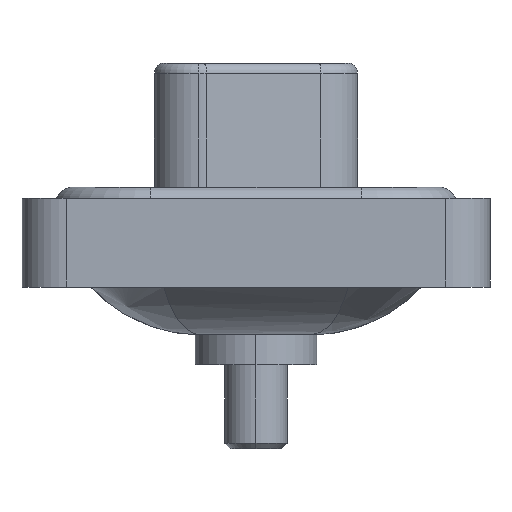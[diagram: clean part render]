
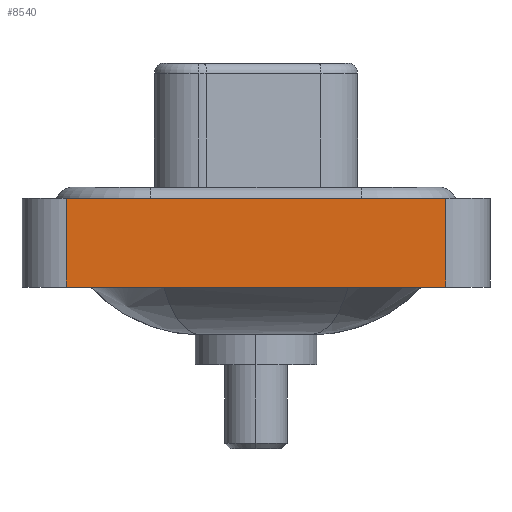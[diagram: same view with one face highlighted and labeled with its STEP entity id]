
A CAD part, left-side view. The second image highlights one B-rep face of the part: STEP entity #8540.
In plain terms, the highlighted planar face has unit normal (-1, 0, 0).
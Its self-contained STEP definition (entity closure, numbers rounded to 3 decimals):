
#223 = EDGE_LOOP ( 'NONE', ( #12306, #4261, #14064, #13628 ) ) ;
#631 = DIRECTION ( 'NONE',  ( 0., 0., 1. ) ) ;
#706 = CARTESIAN_POINT ( 'NONE',  ( -7.3, -8.55, -3.6 ) ) ;
#1344 = VECTOR ( 'NONE', #3159, 1000. ) ;
#1601 = EDGE_CURVE ( 'NONE', #3124, #5176, #15187, .T. ) ;
#1877 = DIRECTION ( 'NONE',  ( -1., 0., 0. ) ) ;
#2962 = DIRECTION ( 'NONE',  ( 0., 0., 1. ) ) ;
#3022 = VERTEX_POINT ( 'NONE', #6699 ) ;
#3061 = LINE ( 'NONE', #12001, #14395 ) ;
#3124 = VERTEX_POINT ( 'NONE', #13640 ) ;
#3159 = DIRECTION ( 'NONE',  ( 0., -1., 0. ) ) ;
#3712 = LINE ( 'NONE', #12402, #6474 ) ;
#4261 = ORIENTED_EDGE ( 'NONE', *, *, #7239, .F. ) ;
#4659 = CARTESIAN_POINT ( 'NONE',  ( -7.3, -8.55, -3.6 ) ) ;
#5176 = VERTEX_POINT ( 'NONE', #16100 ) ;
#6334 = CARTESIAN_POINT ( 'NONE',  ( -7.3, -8.55, -3.6 ) ) ;
#6474 = VECTOR ( 'NONE', #13800, 1000. ) ;
#6487 = AXIS2_PLACEMENT_3D ( 'NONE', #706, #1877, #2962 ) ;
#6699 = CARTESIAN_POINT ( 'NONE',  ( -7.3, 8.55, -3.6 ) ) ;
#7047 = EDGE_CURVE ( 'NONE', #3022, #8860, #3061, .T. ) ;
#7239 = EDGE_CURVE ( 'NONE', #8860, #5176, #3712, .T. ) ;
#7329 = VECTOR ( 'NONE', #12937, 1000. ) ;
#8540 = ADVANCED_FACE ( 'NONE', ( #9445 ), #9602, .T. ) ;
#8860 = VERTEX_POINT ( 'NONE', #12478 ) ;
#9445 = FACE_OUTER_BOUND ( 'NONE', #223, .T. ) ;
#9602 = PLANE ( 'NONE',  #6487 ) ;
#12001 = CARTESIAN_POINT ( 'NONE',  ( -7.3, 8.55, -3.6 ) ) ;
#12306 = ORIENTED_EDGE ( 'NONE', *, *, #1601, .T. ) ;
#12402 = CARTESIAN_POINT ( 'NONE',  ( -7.3, -8.55, 0.4 ) ) ;
#12478 = CARTESIAN_POINT ( 'NONE',  ( -7.3, 8.55, 0.4 ) ) ;
#12937 = DIRECTION ( 'NONE',  ( 0., 0., 1. ) ) ;
#13628 = ORIENTED_EDGE ( 'NONE', *, *, #15407, .T. ) ;
#13640 = CARTESIAN_POINT ( 'NONE',  ( -7.3, -8.55, -3.6 ) ) ;
#13800 = DIRECTION ( 'NONE',  ( 0., -1., 0. ) ) ;
#14064 = ORIENTED_EDGE ( 'NONE', *, *, #7047, .F. ) ;
#14395 = VECTOR ( 'NONE', #631, 1000. ) ;
#15187 = LINE ( 'NONE', #6334, #7329 ) ;
#15407 = EDGE_CURVE ( 'NONE', #3022, #3124, #16081, .T. ) ;
#16081 = LINE ( 'NONE', #4659, #1344 ) ;
#16100 = CARTESIAN_POINT ( 'NONE',  ( -7.3, -8.55, 0.4 ) ) ;
